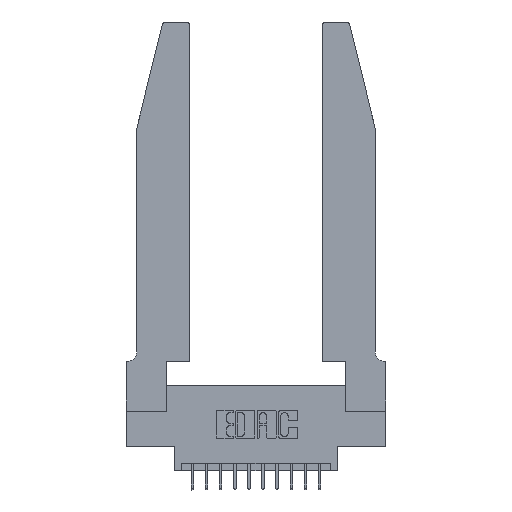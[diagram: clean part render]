
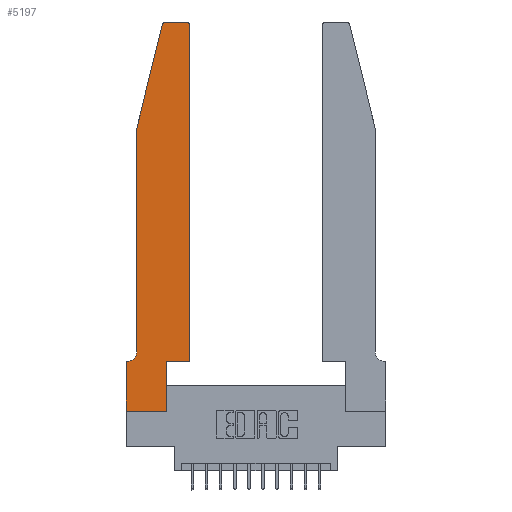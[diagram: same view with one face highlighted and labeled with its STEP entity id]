
A CAD part, top view. The second image highlights one B-rep face of the part: STEP entity #5197.
In plain terms, the highlighted planar face has unit normal (0, 0, 1).
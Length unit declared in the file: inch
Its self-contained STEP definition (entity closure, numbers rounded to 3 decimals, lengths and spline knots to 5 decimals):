
#124 = VERTEX_POINT ( 'NONE', #16938 ) ;
#195 = CIRCLE ( 'NONE', #17077, 0.07 ) ;
#249 = DIRECTION ( 'NONE',  ( 0., -1., 0. ) ) ;
#591 = CARTESIAN_POINT ( 'NONE',  ( 0.0755, 2., 0.37 ) ) ;
#1185 = VERTEX_POINT ( 'NONE', #591 ) ;
#1565 = EDGE_CURVE ( 'NONE', #14302, #11874, #9709, .T. ) ;
#1701 = CARTESIAN_POINT ( 'NONE',  ( 0., 0.35, 0.37 ) ) ;
#1867 = CARTESIAN_POINT ( 'NONE',  ( 0.2865, 0.35, 0.37 ) ) ;
#1878 = VECTOR ( 'NONE', #15028, 39.37008 ) ;
#2212 = ORIENTED_EDGE ( 'NONE', *, *, #7880, .T. ) ;
#2854 = CIRCLE ( 'NONE', #12599, 0.03 ) ;
#2977 = VERTEX_POINT ( 'NONE', #12425 ) ;
#3019 = EDGE_CURVE ( 'NONE', #15189, #1185, #7221, .T. ) ;
#3070 = CARTESIAN_POINT ( 'NONE',  ( 0.0755, 0.35, 0.37 ) ) ;
#3342 = DIRECTION ( 'NONE',  ( -1., 0., 0. ) ) ;
#3542 = EDGE_CURVE ( 'NONE', #11268, #124, #7263, .T. ) ;
#3545 = CIRCLE ( 'NONE', #9776, 0.03 ) ;
#4282 = VERTEX_POINT ( 'NONE', #8156 ) ;
#4289 = LINE ( 'NONE', #3070, #9893 ) ;
#4471 = DIRECTION ( 'NONE',  ( 1., 0., 0. ) ) ;
#4639 = LINE ( 'NONE', #16394, #15996 ) ;
#4819 = EDGE_CURVE ( 'NONE', #1185, #16974, #9914, .T. ) ;
#5197 = ADVANCED_FACE ( 'NONE', ( #6365 ), #10297, .T. ) ;
#5310 = DIRECTION ( 'NONE',  ( 0., 0., 1. ) ) ;
#5798 = LINE ( 'NONE', #1867, #10989 ) ;
#5889 = DIRECTION ( 'NONE',  ( -0.239, -0.971, 0. ) ) ;
#6149 = DIRECTION ( 'NONE',  ( 0., 0., -1. ) ) ;
#6263 = DIRECTION ( 'NONE',  ( -1., 0., 0. ) ) ;
#6365 = FACE_OUTER_BOUND ( 'NONE', #12867, .T. ) ;
#6683 = ORIENTED_EDGE ( 'NONE', *, *, #1565, .T. ) ;
#6778 = VERTEX_POINT ( 'NONE', #12403 ) ;
#7072 = EDGE_CURVE ( 'NONE', #6778, #14302, #4289, .T. ) ;
#7188 = VECTOR ( 'NONE', #6263, 39.37008 ) ;
#7221 = LINE ( 'NONE', #12525, #10030 ) ;
#7240 = CARTESIAN_POINT ( 'NONE',  ( 0.0055, 0.42, 0.37 ) ) ;
#7263 = LINE ( 'NONE', #8818, #7188 ) ;
#7331 = ORIENTED_EDGE ( 'NONE', *, *, #14102, .T. ) ;
#7481 = CARTESIAN_POINT ( 'NONE',  ( 0., 0., 0.37 ) ) ;
#7856 = ORIENTED_EDGE ( 'NONE', *, *, #14326, .T. ) ;
#7880 = EDGE_CURVE ( 'NONE', #124, #15189, #3545, .T. ) ;
#7968 = CARTESIAN_POINT ( 'NONE',  ( 0., 0.35, 0.37 ) ) ;
#8086 = DIRECTION ( 'NONE',  ( 0., 0., 1. ) ) ;
#8156 = CARTESIAN_POINT ( 'NONE',  ( 0.4505, 0.35, 0.37 ) ) ;
#8296 = ORIENTED_EDGE ( 'NONE', *, *, #13486, .T. ) ;
#8531 = CARTESIAN_POINT ( 'NONE',  ( 0.2865, 0.35, 0.37 ) ) ;
#8553 = EDGE_CURVE ( 'NONE', #2977, #11268, #2854, .T. ) ;
#8576 = CARTESIAN_POINT ( 'NONE',  ( 0., 0., 0.37 ) ) ;
#8698 = DIRECTION ( 'NONE',  ( 0., 1., 0. ) ) ;
#8818 = CARTESIAN_POINT ( 'NONE',  ( 0.2605, 2.75, 0.37 ) ) ;
#9060 = DIRECTION ( 'NONE',  ( 1., 0., 0. ) ) ;
#9666 = DIRECTION ( 'NONE',  ( -1., 0., 0. ) ) ;
#9709 = LINE ( 'NONE', #8576, #11225 ) ;
#9776 = AXIS2_PLACEMENT_3D ( 'NONE', #11505, #10114, #9060 ) ;
#9893 = VECTOR ( 'NONE', #9666, 39.37008 ) ;
#9914 = LINE ( 'NONE', #15011, #11961 ) ;
#9987 = LINE ( 'NONE', #12836, #14877 ) ;
#10030 = VECTOR ( 'NONE', #5889, 39.37008 ) ;
#10114 = DIRECTION ( 'NONE',  ( 0., 0., 1. ) ) ;
#10297 = PLANE ( 'NONE',  #10896 ) ;
#10833 = DIRECTION ( 'NONE',  ( 0., -1., 0. ) ) ;
#10867 = CARTESIAN_POINT ( 'NONE',  ( 0.4205, 2.72, 0.37 ) ) ;
#10896 = AXIS2_PLACEMENT_3D ( 'NONE', #7968, #5310, #15658 ) ;
#10935 = ORIENTED_EDGE ( 'NONE', *, *, #4819, .T. ) ;
#10989 = VECTOR ( 'NONE', #13910, 39.37008 ) ;
#11225 = VECTOR ( 'NONE', #10833, 39.37008 ) ;
#11226 = LINE ( 'NONE', #16491, #1878 ) ;
#11268 = VERTEX_POINT ( 'NONE', #16485 ) ;
#11505 = CARTESIAN_POINT ( 'NONE',  ( 0.284, 2.72, 0.37 ) ) ;
#11517 = ORIENTED_EDGE ( 'NONE', *, *, #12111, .T. ) ;
#11874 = VERTEX_POINT ( 'NONE', #7481 ) ;
#11891 = CARTESIAN_POINT ( 'NONE',  ( 0.2865, 0., 0.37 ) ) ;
#11961 = VECTOR ( 'NONE', #249, 39.37008 ) ;
#12111 = EDGE_CURVE ( 'NONE', #16666, #16808, #5798, .T. ) ;
#12294 = ORIENTED_EDGE ( 'NONE', *, *, #16574, .T. ) ;
#12403 = CARTESIAN_POINT ( 'NONE',  ( 0.0055, 0.35, 0.37 ) ) ;
#12425 = CARTESIAN_POINT ( 'NONE',  ( 0.4505, 2.72, 0.37 ) ) ;
#12525 = CARTESIAN_POINT ( 'NONE',  ( 0.0755, 2., 0.37 ) ) ;
#12599 = AXIS2_PLACEMENT_3D ( 'NONE', #10867, #8086, #13462 ) ;
#12645 = ORIENTED_EDGE ( 'NONE', *, *, #3019, .T. ) ;
#12836 = CARTESIAN_POINT ( 'NONE',  ( 0.4505, 0.35, 0.37 ) ) ;
#12867 = EDGE_LOOP ( 'NONE', ( #14100, #2212, #12645, #10935, #7331, #13958, #6683, #7856, #11517, #12294, #8296, #17064 ) ) ;
#13462 = DIRECTION ( 'NONE',  ( 1., 0., 0. ) ) ;
#13486 = EDGE_CURVE ( 'NONE', #4282, #2977, #9987, .T. ) ;
#13910 = DIRECTION ( 'NONE',  ( 0., 1., 0. ) ) ;
#13958 = ORIENTED_EDGE ( 'NONE', *, *, #7072, .T. ) ;
#14035 = CARTESIAN_POINT ( 'NONE',  ( 0.25487, 2.72718, 0.37 ) ) ;
#14100 = ORIENTED_EDGE ( 'NONE', *, *, #3542, .T. ) ;
#14102 = EDGE_CURVE ( 'NONE', #16974, #6778, #195, .T. ) ;
#14302 = VERTEX_POINT ( 'NONE', #1701 ) ;
#14326 = EDGE_CURVE ( 'NONE', #11874, #16666, #4639, .T. ) ;
#14877 = VECTOR ( 'NONE', #8698, 39.37008 ) ;
#15011 = CARTESIAN_POINT ( 'NONE',  ( 0.0755, 2., 0.37 ) ) ;
#15028 = DIRECTION ( 'NONE',  ( 1., 0., 0. ) ) ;
#15189 = VERTEX_POINT ( 'NONE', #14035 ) ;
#15658 = DIRECTION ( 'NONE',  ( 1., 0., 0. ) ) ;
#15996 = VECTOR ( 'NONE', #4471, 39.37008 ) ;
#16023 = CARTESIAN_POINT ( 'NONE',  ( 0.0755, 0.42, 0.37 ) ) ;
#16394 = CARTESIAN_POINT ( 'NONE',  ( 0., 0., 0.37 ) ) ;
#16485 = CARTESIAN_POINT ( 'NONE',  ( 0.4205, 2.75, 0.37 ) ) ;
#16491 = CARTESIAN_POINT ( 'NONE',  ( 0.4505, 0.35, 0.37 ) ) ;
#16574 = EDGE_CURVE ( 'NONE', #16808, #4282, #11226, .T. ) ;
#16666 = VERTEX_POINT ( 'NONE', #11891 ) ;
#16808 = VERTEX_POINT ( 'NONE', #8531 ) ;
#16938 = CARTESIAN_POINT ( 'NONE',  ( 0.284, 2.75, 0.37 ) ) ;
#16974 = VERTEX_POINT ( 'NONE', #16023 ) ;
#17064 = ORIENTED_EDGE ( 'NONE', *, *, #8553, .T. ) ;
#17077 = AXIS2_PLACEMENT_3D ( 'NONE', #7240, #6149, #3342 ) ;
